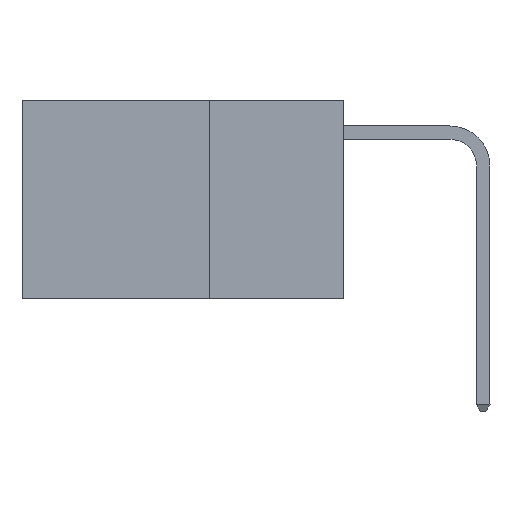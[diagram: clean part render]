
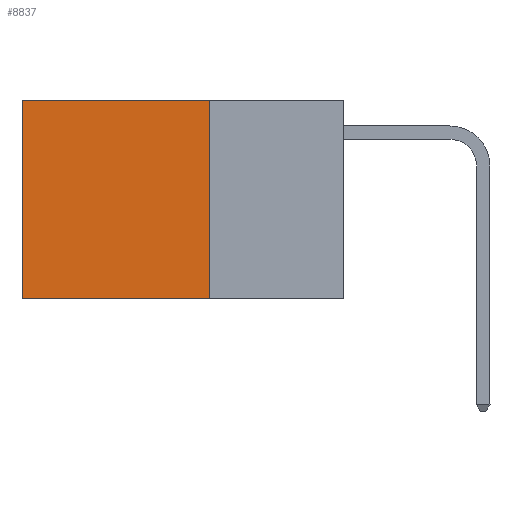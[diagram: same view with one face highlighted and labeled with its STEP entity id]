
A CAD part, left-side view. The second image highlights one B-rep face of the part: STEP entity #8837.
In plain terms, the highlighted planar face has unit normal (-1, 0, 0).
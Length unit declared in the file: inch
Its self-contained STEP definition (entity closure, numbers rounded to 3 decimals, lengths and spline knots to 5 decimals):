
#224 = CARTESIAN_POINT ( 'NONE',  ( 0.2625, 0.6, 0. ) ) ;
#1553 = LINE ( 'NONE', #10226, #10807 ) ;
#3586 = VECTOR ( 'NONE', #6926, 39.37008 ) ;
#4404 = CARTESIAN_POINT ( 'NONE',  ( 0.2625, 0.25, 0. ) ) ;
#4789 = DIRECTION ( 'NONE',  ( 0., 1., 0. ) ) ;
#6175 = EDGE_CURVE ( 'NONE', #18454, #18359, #1553, .T. ) ;
#6735 = CARTESIAN_POINT ( 'NONE',  ( 0.2625, 0.25, 0. ) ) ;
#6926 = DIRECTION ( 'NONE',  ( 0., 0., -1. ) ) ;
#7271 = DIRECTION ( 'NONE',  ( 1., 0., 0. ) ) ;
#7482 = ORIENTED_EDGE ( 'NONE', *, *, #6175, .F. ) ;
#7674 = ORIENTED_EDGE ( 'NONE', *, *, #16389, .T. ) ;
#8433 = VERTEX_POINT ( 'NONE', #8907 ) ;
#8671 = PLANE ( 'NONE',  #12265 ) ;
#8837 = ADVANCED_FACE ( 'NONE', ( #14817 ), #8671, .F. ) ;
#8866 = EDGE_LOOP ( 'NONE', ( #7674, #7482, #18803, #10867 ) ) ;
#8907 = CARTESIAN_POINT ( 'NONE',  ( 0.2625, 0.6, 0. ) ) ;
#8992 = DIRECTION ( 'NONE',  ( 0., 0., -1. ) ) ;
#9600 = VERTEX_POINT ( 'NONE', #6735 ) ;
#10226 = CARTESIAN_POINT ( 'NONE',  ( 0.2625, 0.25, -0.37 ) ) ;
#10264 = EDGE_CURVE ( 'NONE', #9600, #8433, #16967, .T. ) ;
#10807 = VECTOR ( 'NONE', #16359, 39.37008 ) ;
#10867 = ORIENTED_EDGE ( 'NONE', *, *, #10264, .T. ) ;
#12265 = AXIS2_PLACEMENT_3D ( 'NONE', #4404, #7271, #8992 ) ;
#12777 = EDGE_CURVE ( 'NONE', #9600, #18454, #19056, .T. ) ;
#14154 = VECTOR ( 'NONE', #17790, 39.37008 ) ;
#14284 = CARTESIAN_POINT ( 'NONE',  ( 0.2625, 0.25, -0.37 ) ) ;
#14495 = VECTOR ( 'NONE', #4789, 39.37008 ) ;
#14817 = FACE_OUTER_BOUND ( 'NONE', #8866, .T. ) ;
#15467 = CARTESIAN_POINT ( 'NONE',  ( 0.2625, 0.6, -0.37 ) ) ;
#16359 = DIRECTION ( 'NONE',  ( 0., 1., 0. ) ) ;
#16389 = EDGE_CURVE ( 'NONE', #8433, #18359, #17883, .T. ) ;
#16967 = LINE ( 'NONE', #18372, #14495 ) ;
#17606 = CARTESIAN_POINT ( 'NONE',  ( 0.2625, 0.25, 0. ) ) ;
#17790 = DIRECTION ( 'NONE',  ( 0., 0., -1. ) ) ;
#17883 = LINE ( 'NONE', #224, #14154 ) ;
#18359 = VERTEX_POINT ( 'NONE', #15467 ) ;
#18372 = CARTESIAN_POINT ( 'NONE',  ( 0.2625, 0.25, 0. ) ) ;
#18454 = VERTEX_POINT ( 'NONE', #14284 ) ;
#18803 = ORIENTED_EDGE ( 'NONE', *, *, #12777, .F. ) ;
#19056 = LINE ( 'NONE', #17606, #3586 ) ;
